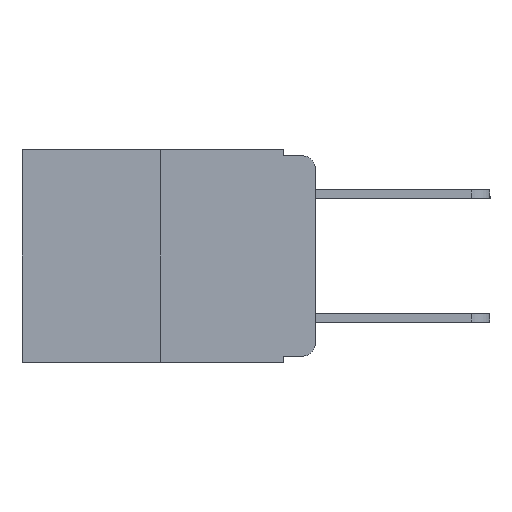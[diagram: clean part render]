
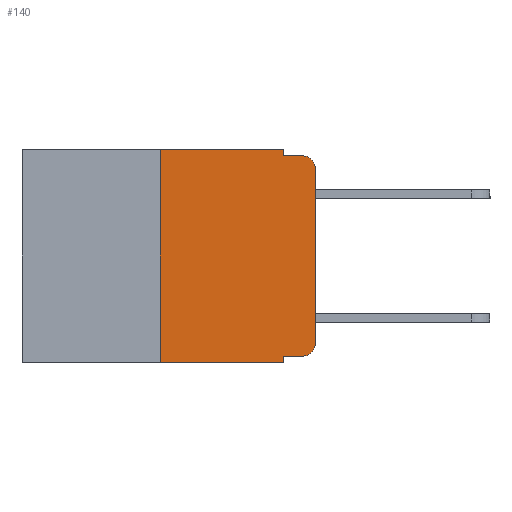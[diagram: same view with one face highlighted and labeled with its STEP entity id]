
A CAD part, left-side view. The second image highlights one B-rep face of the part: STEP entity #140.
In plain terms, the highlighted planar face has unit normal (-1, 0, 0).
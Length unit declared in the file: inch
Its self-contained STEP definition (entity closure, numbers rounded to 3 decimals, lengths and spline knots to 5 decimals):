
#83 = LINE ( 'NONE', #10475, #2808 ) ;
#140 = ADVANCED_FACE ( 'NONE', ( #3813 ), #10764, .F. ) ;
#218 = EDGE_CURVE ( 'NONE', #3861, #5959, #4605, .T. ) ;
#239 = CARTESIAN_POINT ( 'NONE',  ( 0., 0., -0.03 ) ) ;
#296 = VERTEX_POINT ( 'NONE', #8343 ) ;
#347 = EDGE_CURVE ( 'NONE', #6545, #1068, #9893, .T. ) ;
#364 = VERTEX_POINT ( 'NONE', #5064 ) ;
#519 = DIRECTION ( 'NONE',  ( -1., 0., 0. ) ) ;
#557 = EDGE_CURVE ( 'NONE', #5959, #3752, #6027, .T. ) ;
#621 = VERTEX_POINT ( 'NONE', #11100 ) ;
#1068 = VERTEX_POINT ( 'NONE', #4126 ) ;
#1780 = VERTEX_POINT ( 'NONE', #10776 ) ;
#2028 = VECTOR ( 'NONE', #9012, 39.37008 ) ;
#2147 = VERTEX_POINT ( 'NONE', #7296 ) ;
#2327 = CARTESIAN_POINT ( 'NONE',  ( 0., 0.02, -0.313 ) ) ;
#2756 = EDGE_CURVE ( 'NONE', #621, #1780, #7786, .T. ) ;
#2808 = VECTOR ( 'NONE', #10459, 39.37008 ) ;
#2969 = EDGE_CURVE ( 'NONE', #1780, #3861, #11435, .T. ) ;
#2998 = CARTESIAN_POINT ( 'NONE',  ( 0., 0.25, 0. ) ) ;
#3066 = AXIS2_PLACEMENT_3D ( 'NONE', #10557, #3114, #11071 ) ;
#3114 = DIRECTION ( 'NONE',  ( -1., 0., 0. ) ) ;
#3302 = VECTOR ( 'NONE', #7456, 39.37008 ) ;
#3395 = EDGE_CURVE ( 'NONE', #2147, #364, #9937, .T. ) ;
#3752 = VERTEX_POINT ( 'NONE', #8139 ) ;
#3813 = FACE_OUTER_BOUND ( 'NONE', #7512, .T. ) ;
#3861 = VERTEX_POINT ( 'NONE', #6660 ) ;
#4126 = CARTESIAN_POINT ( 'NONE',  ( 0., 0.051, -0.01 ) ) ;
#4605 = LINE ( 'NONE', #11533, #6982 ) ;
#4692 = CARTESIAN_POINT ( 'NONE',  ( 0., 0.051, 0. ) ) ;
#4837 = LINE ( 'NONE', #10911, #2028 ) ;
#5064 = CARTESIAN_POINT ( 'NONE',  ( 0., 0.25, 0. ) ) ;
#5558 = AXIS2_PLACEMENT_3D ( 'NONE', #10663, #9271, #10099 ) ;
#5566 = VECTOR ( 'NONE', #8218, 39.37008 ) ;
#5959 = VERTEX_POINT ( 'NONE', #239 ) ;
#5997 = ORIENTED_EDGE ( 'NONE', *, *, #218, .T. ) ;
#6027 = CIRCLE ( 'NONE', #3066, 0.02 ) ;
#6092 = DIRECTION ( 'NONE',  ( 0., 0., 1. ) ) ;
#6171 = EDGE_CURVE ( 'NONE', #1068, #3752, #4837, .T. ) ;
#6237 = DIRECTION ( 'NONE',  ( 0., 0., -1. ) ) ;
#6246 = DIRECTION ( 'NONE',  ( 0., 0., -1. ) ) ;
#6384 = VECTOR ( 'NONE', #6246, 39.37008 ) ;
#6545 = VERTEX_POINT ( 'NONE', #7032 ) ;
#6651 = LINE ( 'NONE', #9475, #6384 ) ;
#6660 = CARTESIAN_POINT ( 'NONE',  ( 0., 0., -0.313 ) ) ;
#6982 = VECTOR ( 'NONE', #6092, 39.37008 ) ;
#7032 = CARTESIAN_POINT ( 'NONE',  ( 0., 0.051, 0. ) ) ;
#7137 = CARTESIAN_POINT ( 'NONE',  ( 0., 0.473, 0. ) ) ;
#7180 = ORIENTED_EDGE ( 'NONE', *, *, #2969, .T. ) ;
#7229 = ORIENTED_EDGE ( 'NONE', *, *, #2756, .T. ) ;
#7296 = CARTESIAN_POINT ( 'NONE',  ( 0., 0.25, -0.343 ) ) ;
#7456 = DIRECTION ( 'NONE',  ( 0., -1., 0. ) ) ;
#7512 = EDGE_LOOP ( 'NONE', ( #5997, #9538, #9441, #9332, #9096, #8899, #7710, #7523, #7229, #7180 ) ) ;
#7523 = ORIENTED_EDGE ( 'NONE', *, *, #11585, .F. ) ;
#7710 = ORIENTED_EDGE ( 'NONE', *, *, #10799, .T. ) ;
#7786 = LINE ( 'NONE', #8629, #5566 ) ;
#8068 = LINE ( 'NONE', #7137, #3302 ) ;
#8088 = VECTOR ( 'NONE', #6237, 39.37008 ) ;
#8139 = CARTESIAN_POINT ( 'NONE',  ( 0., 0.02, -0.01 ) ) ;
#8218 = DIRECTION ( 'NONE',  ( 0., -1., 0. ) ) ;
#8343 = CARTESIAN_POINT ( 'NONE',  ( 0., 0.051, -0.343 ) ) ;
#8629 = CARTESIAN_POINT ( 'NONE',  ( 0., 0.051, -0.333 ) ) ;
#8784 = AXIS2_PLACEMENT_3D ( 'NONE', #2327, #519, #11324 ) ;
#8899 = ORIENTED_EDGE ( 'NONE', *, *, #3395, .F. ) ;
#9012 = DIRECTION ( 'NONE',  ( 0., -1., 0. ) ) ;
#9096 = ORIENTED_EDGE ( 'NONE', *, *, #10521, .F. ) ;
#9271 = DIRECTION ( 'NONE',  ( 1., 0., 0. ) ) ;
#9332 = ORIENTED_EDGE ( 'NONE', *, *, #347, .F. ) ;
#9441 = ORIENTED_EDGE ( 'NONE', *, *, #6171, .F. ) ;
#9475 = CARTESIAN_POINT ( 'NONE',  ( 0., 0.051, 0. ) ) ;
#9538 = ORIENTED_EDGE ( 'NONE', *, *, #557, .T. ) ;
#9893 = LINE ( 'NONE', #4692, #8088 ) ;
#9937 = LINE ( 'NONE', #2998, #10975 ) ;
#10099 = DIRECTION ( 'NONE',  ( 0., 0., -1. ) ) ;
#10459 = DIRECTION ( 'NONE',  ( 0., -1., 0. ) ) ;
#10475 = CARTESIAN_POINT ( 'NONE',  ( 0., 0.473, -0.343 ) ) ;
#10521 = EDGE_CURVE ( 'NONE', #364, #6545, #8068, .T. ) ;
#10557 = CARTESIAN_POINT ( 'NONE',  ( 0., 0.02, -0.03 ) ) ;
#10663 = CARTESIAN_POINT ( 'NONE',  ( 0., 0.473, 0. ) ) ;
#10764 = PLANE ( 'NONE',  #5558 ) ;
#10776 = CARTESIAN_POINT ( 'NONE',  ( 0., 0.02, -0.333 ) ) ;
#10799 = EDGE_CURVE ( 'NONE', #2147, #296, #83, .T. ) ;
#10911 = CARTESIAN_POINT ( 'NONE',  ( 0., 0.051, -0.01 ) ) ;
#10975 = VECTOR ( 'NONE', #11059, 39.37008 ) ;
#11059 = DIRECTION ( 'NONE',  ( 0., 0., 1. ) ) ;
#11071 = DIRECTION ( 'NONE',  ( 0., 0., -1. ) ) ;
#11100 = CARTESIAN_POINT ( 'NONE',  ( 0., 0.051, -0.333 ) ) ;
#11324 = DIRECTION ( 'NONE',  ( 0., 0., -1. ) ) ;
#11435 = CIRCLE ( 'NONE', #8784, 0.02 ) ;
#11533 = CARTESIAN_POINT ( 'NONE',  ( 0., 0., 0. ) ) ;
#11585 = EDGE_CURVE ( 'NONE', #621, #296, #6651, .T. ) ;
